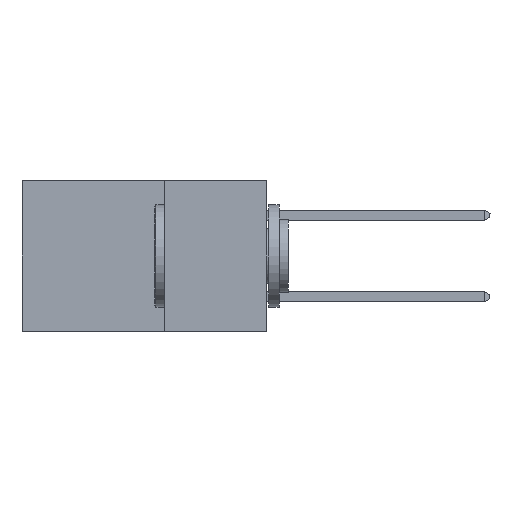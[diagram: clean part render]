
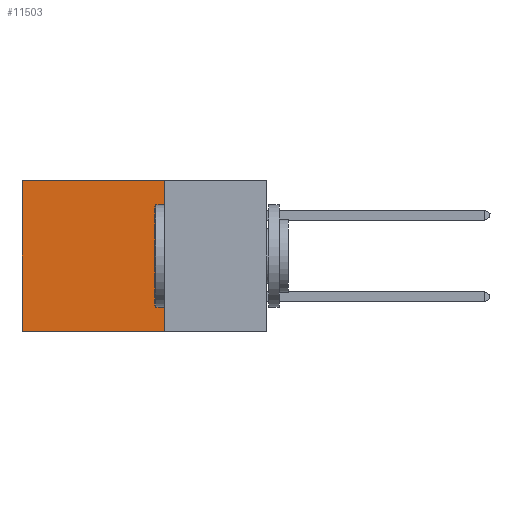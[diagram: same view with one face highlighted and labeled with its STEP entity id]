
A CAD part, left-side view. The second image highlights one B-rep face of the part: STEP entity #11503.
In plain terms, the highlighted planar face has unit normal (-1, 0, 0).
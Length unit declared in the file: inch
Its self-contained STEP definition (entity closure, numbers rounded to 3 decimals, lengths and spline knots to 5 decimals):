
#2406 = CARTESIAN_POINT ( 'NONE',  ( 0.2875, 0.25, -0.37 ) ) ;
#3174 = FACE_OUTER_BOUND ( 'NONE', #12434, .T. ) ;
#3189 = LINE ( 'NONE', #19474, #23522 ) ;
#3486 = LINE ( 'NONE', #18998, #27903 ) ;
#3762 = DIRECTION ( 'NONE',  ( 0., 0., -1. ) ) ;
#3834 = EDGE_CURVE ( 'NONE', #12079, #18735, #28234, .T. ) ;
#4424 = EDGE_CURVE ( 'NONE', #19245, #4639, #3189, .T. ) ;
#4639 = VERTEX_POINT ( 'NONE', #19832 ) ;
#4672 = AXIS2_PLACEMENT_3D ( 'NONE', #5676, #10132, #3762 ) ;
#5676 = CARTESIAN_POINT ( 'NONE',  ( 0.2875, 0.25, 0. ) ) ;
#6647 = CARTESIAN_POINT ( 'NONE',  ( 0.2875, 0.25, 0. ) ) ;
#6794 = CARTESIAN_POINT ( 'NONE',  ( 0.2875, 0.25, 0. ) ) ;
#8560 = DIRECTION ( 'NONE',  ( 0., 1., 0. ) ) ;
#9052 = CARTESIAN_POINT ( 'NONE',  ( 0.2875, 0.6, 0. ) ) ;
#10132 = DIRECTION ( 'NONE',  ( 1., 0., 0. ) ) ;
#10365 = VECTOR ( 'NONE', #17546, 39.37008 ) ;
#11503 = ADVANCED_FACE ( 'NONE', ( #3174 ), #26319, .F. ) ;
#12079 = VERTEX_POINT ( 'NONE', #6794 ) ;
#12434 = EDGE_LOOP ( 'NONE', ( #27217, #18615, #19602, #20427 ) ) ;
#13564 = DIRECTION ( 'NONE',  ( 0., 1., 0. ) ) ;
#16812 = EDGE_CURVE ( 'NONE', #12079, #19245, #3486, .T. ) ;
#17546 = DIRECTION ( 'NONE',  ( 0., 0., -1. ) ) ;
#18615 = ORIENTED_EDGE ( 'NONE', *, *, #22890, .F. ) ;
#18735 = VERTEX_POINT ( 'NONE', #27102 ) ;
#18998 = CARTESIAN_POINT ( 'NONE',  ( 0.2875, 0.25, 0. ) ) ;
#19245 = VERTEX_POINT ( 'NONE', #9052 ) ;
#19474 = CARTESIAN_POINT ( 'NONE',  ( 0.2875, 0.6, 0. ) ) ;
#19602 = ORIENTED_EDGE ( 'NONE', *, *, #3834, .F. ) ;
#19832 = CARTESIAN_POINT ( 'NONE',  ( 0.2875, 0.6, -0.37 ) ) ;
#20427 = ORIENTED_EDGE ( 'NONE', *, *, #16812, .T. ) ;
#22890 = EDGE_CURVE ( 'NONE', #18735, #4639, #23359, .T. ) ;
#23359 = LINE ( 'NONE', #2406, #26073 ) ;
#23522 = VECTOR ( 'NONE', #23825, 39.37008 ) ;
#23825 = DIRECTION ( 'NONE',  ( 0., 0., -1. ) ) ;
#26073 = VECTOR ( 'NONE', #13564, 39.37008 ) ;
#26319 = PLANE ( 'NONE',  #4672 ) ;
#27102 = CARTESIAN_POINT ( 'NONE',  ( 0.2875, 0.25, -0.37 ) ) ;
#27217 = ORIENTED_EDGE ( 'NONE', *, *, #4424, .T. ) ;
#27903 = VECTOR ( 'NONE', #8560, 39.37008 ) ;
#28234 = LINE ( 'NONE', #6647, #10365 ) ;
